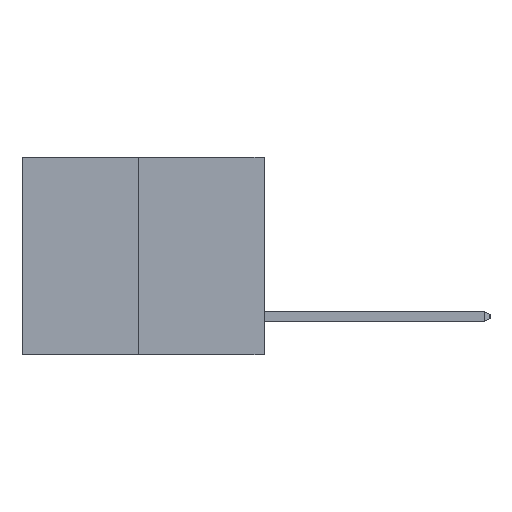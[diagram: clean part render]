
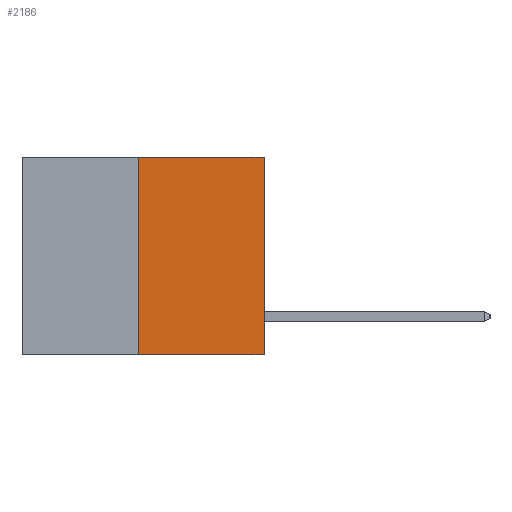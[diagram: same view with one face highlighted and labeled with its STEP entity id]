
A CAD part, left-side view. The second image highlights one B-rep face of the part: STEP entity #2186.
In plain terms, the highlighted planar face has unit normal (-1, 0, 0).
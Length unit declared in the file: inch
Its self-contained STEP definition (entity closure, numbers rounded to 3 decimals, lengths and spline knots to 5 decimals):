
#361 = FACE_OUTER_BOUND ( 'NONE', #13785, .T. ) ;
#585 = VERTEX_POINT ( 'NONE', #13303 ) ;
#1171 = DIRECTION ( 'NONE',  ( 0., -1., 0. ) ) ;
#1353 = DIRECTION ( 'NONE',  ( 0., 0., 1. ) ) ;
#1457 = EDGE_CURVE ( 'NONE', #585, #13210, #12429, .T. ) ;
#2186 = ADVANCED_FACE ( 'NONE', ( #361 ), #5377, .F. ) ;
#2214 = CARTESIAN_POINT ( 'NONE',  ( 0., 0.6, 0. ) ) ;
#2584 = CARTESIAN_POINT ( 'NONE',  ( 0., 0., -0.49 ) ) ;
#3143 = CARTESIAN_POINT ( 'NONE',  ( 0., 0.6, -0.49 ) ) ;
#3665 = ORIENTED_EDGE ( 'NONE', *, *, #1457, .F. ) ;
#3739 = CARTESIAN_POINT ( 'NONE',  ( 0., 0.312, -0.49 ) ) ;
#3748 = VECTOR ( 'NONE', #1353, 39.37008 ) ;
#4444 = DIRECTION ( 'NONE',  ( 0., 0., -1. ) ) ;
#4581 = CARTESIAN_POINT ( 'NONE',  ( 0., 0., 0. ) ) ;
#4901 = VECTOR ( 'NONE', #9367, 39.37008 ) ;
#5377 = PLANE ( 'NONE',  #11335 ) ;
#5458 = VERTEX_POINT ( 'NONE', #2584 ) ;
#6026 = VERTEX_POINT ( 'NONE', #3739 ) ;
#6372 = DIRECTION ( 'NONE',  ( 0., -1., 0. ) ) ;
#7365 = EDGE_CURVE ( 'NONE', #6026, #585, #7729, .T. ) ;
#7498 = EDGE_CURVE ( 'NONE', #5458, #13210, #10920, .T. ) ;
#7602 = CARTESIAN_POINT ( 'NONE',  ( 0., 0.6, 0. ) ) ;
#7729 = LINE ( 'NONE', #10401, #4901 ) ;
#8610 = DIRECTION ( 'NONE',  ( 1., 0., 0. ) ) ;
#9367 = DIRECTION ( 'NONE',  ( 0., 0., 1. ) ) ;
#9534 = ORIENTED_EDGE ( 'NONE', *, *, #12646, .T. ) ;
#9564 = VECTOR ( 'NONE', #6372, 39.37008 ) ;
#10401 = CARTESIAN_POINT ( 'NONE',  ( 0., 0.312, -0.49 ) ) ;
#10641 = ORIENTED_EDGE ( 'NONE', *, *, #7365, .F. ) ;
#10920 = LINE ( 'NONE', #4581, #3748 ) ;
#11335 = AXIS2_PLACEMENT_3D ( 'NONE', #7602, #8610, #4444 ) ;
#12429 = LINE ( 'NONE', #2214, #9564 ) ;
#12646 = EDGE_CURVE ( 'NONE', #6026, #5458, #12691, .T. ) ;
#12672 = ORIENTED_EDGE ( 'NONE', *, *, #7498, .T. ) ;
#12691 = LINE ( 'NONE', #3143, #13377 ) ;
#13210 = VERTEX_POINT ( 'NONE', #13402 ) ;
#13303 = CARTESIAN_POINT ( 'NONE',  ( 0., 0.312, 0. ) ) ;
#13377 = VECTOR ( 'NONE', #1171, 39.37008 ) ;
#13402 = CARTESIAN_POINT ( 'NONE',  ( 0., 0., 0. ) ) ;
#13785 = EDGE_LOOP ( 'NONE', ( #10641, #9534, #12672, #3665 ) ) ;
